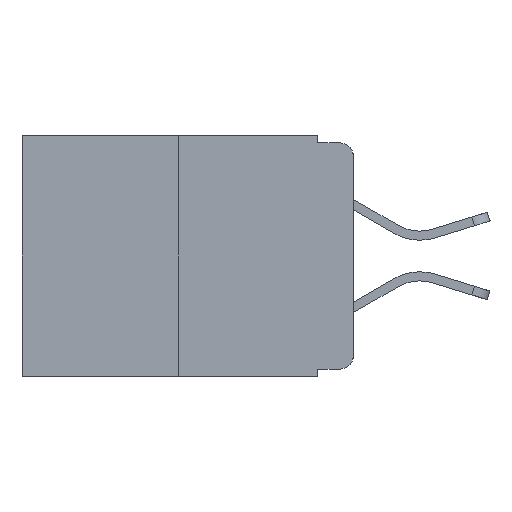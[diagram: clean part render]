
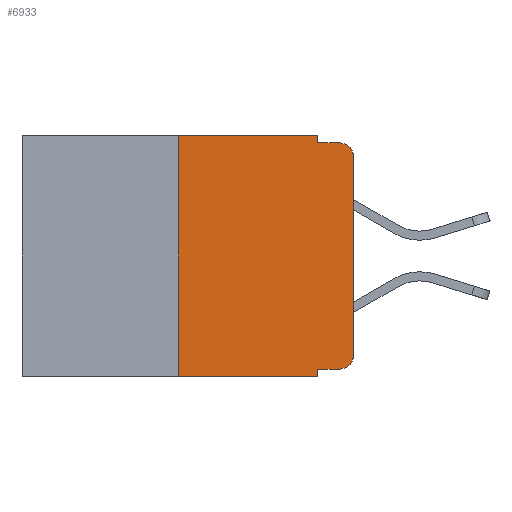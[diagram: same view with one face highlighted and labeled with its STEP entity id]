
A CAD part, left-side view. The second image highlights one B-rep face of the part: STEP entity #6933.
In plain terms, the highlighted planar face has unit normal (-1, 0, 0).
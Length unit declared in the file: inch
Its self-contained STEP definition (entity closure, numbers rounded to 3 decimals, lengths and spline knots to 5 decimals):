
#56 = ORIENTED_EDGE ( 'NONE', *, *, #13089, .T. ) ;
#123 = CARTESIAN_POINT ( 'NONE',  ( 0., 0.051, 0. ) ) ;
#607 = CARTESIAN_POINT ( 'NONE',  ( 0., 0.051, -0.01 ) ) ;
#1297 = VERTEX_POINT ( 'NONE', #15074 ) ;
#1436 = FACE_OUTER_BOUND ( 'NONE', #13858, .T. ) ;
#2048 = EDGE_CURVE ( 'NONE', #14311, #5021, #21147, .T. ) ;
#2507 = ORIENTED_EDGE ( 'NONE', *, *, #4083, .F. ) ;
#2762 = VECTOR ( 'NONE', #11772, 39.37008 ) ;
#3166 = DIRECTION ( 'NONE',  ( 0., -1., 0. ) ) ;
#3186 = EDGE_CURVE ( 'NONE', #1297, #5021, #16227, .T. ) ;
#3219 = ORIENTED_EDGE ( 'NONE', *, *, #9746, .F. ) ;
#3296 = VECTOR ( 'NONE', #3166, 39.37008 ) ;
#3500 = EDGE_CURVE ( 'NONE', #12253, #11377, #20334, .T. ) ;
#3639 = EDGE_CURVE ( 'NONE', #8644, #14191, #11302, .T. ) ;
#3788 = CARTESIAN_POINT ( 'NONE',  ( 0., 0., 0. ) ) ;
#3923 = CARTESIAN_POINT ( 'NONE',  ( 0., 0.051, -0.01 ) ) ;
#4083 = EDGE_CURVE ( 'NONE', #14311, #12253, #13909, .T. ) ;
#4206 = EDGE_CURVE ( 'NONE', #1297, #5745, #5074, .T. ) ;
#4290 = ORIENTED_EDGE ( 'NONE', *, *, #3639, .T. ) ;
#4428 = EDGE_CURVE ( 'NONE', #13529, #14191, #20040, .T. ) ;
#4729 = AXIS2_PLACEMENT_3D ( 'NONE', #18329, #4995, #8584 ) ;
#4995 = DIRECTION ( 'NONE',  ( -1., 0., 0. ) ) ;
#5021 = VERTEX_POINT ( 'NONE', #17077 ) ;
#5074 = LINE ( 'NONE', #17989, #17493 ) ;
#5465 = CARTESIAN_POINT ( 'NONE',  ( 0., 0.02, -0.03 ) ) ;
#5649 = ORIENTED_EDGE ( 'NONE', *, *, #3186, .F. ) ;
#5745 = VERTEX_POINT ( 'NONE', #20886 ) ;
#6933 = ADVANCED_FACE ( 'NONE', ( #1436 ), #10618, .F. ) ;
#6961 = CARTESIAN_POINT ( 'NONE',  ( 0., 0.051, 0. ) ) ;
#6985 = DIRECTION ( 'NONE',  ( 0., 0., 1. ) ) ;
#7328 = CARTESIAN_POINT ( 'NONE',  ( 0., 0.473, -0.343 ) ) ;
#7394 = CIRCLE ( 'NONE', #4729, 0.02 ) ;
#8537 = DIRECTION ( 'NONE',  ( 1., 0., 0. ) ) ;
#8584 = DIRECTION ( 'NONE',  ( 0., 0., -1. ) ) ;
#8644 = VERTEX_POINT ( 'NONE', #13915 ) ;
#9286 = VECTOR ( 'NONE', #10568, 39.37008 ) ;
#9569 = VECTOR ( 'NONE', #6985, 39.37008 ) ;
#9746 = EDGE_CURVE ( 'NONE', #11377, #13529, #17118, .T. ) ;
#10413 = ORIENTED_EDGE ( 'NONE', *, *, #4206, .T. ) ;
#10568 = DIRECTION ( 'NONE',  ( 0., -1., 0. ) ) ;
#10618 = PLANE ( 'NONE',  #13436 ) ;
#11301 = ORIENTED_EDGE ( 'NONE', *, *, #3500, .F. ) ;
#11302 = CIRCLE ( 'NONE', #16244, 0.02 ) ;
#11377 = VERTEX_POINT ( 'NONE', #6961 ) ;
#11388 = VECTOR ( 'NONE', #17624, 39.37008 ) ;
#11772 = DIRECTION ( 'NONE',  ( 0., 0., -1. ) ) ;
#11904 = CARTESIAN_POINT ( 'NONE',  ( 0., 0.02, -0.01 ) ) ;
#12173 = DIRECTION ( 'NONE',  ( 0., -1., 0. ) ) ;
#12253 = VERTEX_POINT ( 'NONE', #14632 ) ;
#12328 = VECTOR ( 'NONE', #19517, 39.37008 ) ;
#12486 = CARTESIAN_POINT ( 'NONE',  ( 0., 0., -0.313 ) ) ;
#12581 = DIRECTION ( 'NONE',  ( -1., 0., 0. ) ) ;
#12709 = CARTESIAN_POINT ( 'NONE',  ( 0., 0.051, 0. ) ) ;
#13089 = EDGE_CURVE ( 'NONE', #5745, #16163, #7394, .T. ) ;
#13268 = DIRECTION ( 'NONE',  ( 0., -1., 0. ) ) ;
#13381 = VECTOR ( 'NONE', #12173, 39.37008 ) ;
#13436 = AXIS2_PLACEMENT_3D ( 'NONE', #16791, #8537, #20093 ) ;
#13529 = VERTEX_POINT ( 'NONE', #3923 ) ;
#13756 = ORIENTED_EDGE ( 'NONE', *, *, #4428, .F. ) ;
#13858 = EDGE_LOOP ( 'NONE', ( #21193, #4290, #13756, #3219, #11301, #2507, #15617, #5649, #10413, #56 ) ) ;
#13909 = LINE ( 'NONE', #16063, #12328 ) ;
#13915 = CARTESIAN_POINT ( 'NONE',  ( 0., 0., -0.03 ) ) ;
#14189 = DIRECTION ( 'NONE',  ( 0., 0., -1. ) ) ;
#14191 = VERTEX_POINT ( 'NONE', #11904 ) ;
#14311 = VERTEX_POINT ( 'NONE', #17654 ) ;
#14632 = CARTESIAN_POINT ( 'NONE',  ( 0., 0.25, 0. ) ) ;
#15074 = CARTESIAN_POINT ( 'NONE',  ( 0., 0.051, -0.333 ) ) ;
#15617 = ORIENTED_EDGE ( 'NONE', *, *, #2048, .T. ) ;
#16063 = CARTESIAN_POINT ( 'NONE',  ( 0., 0.25, 0. ) ) ;
#16163 = VERTEX_POINT ( 'NONE', #12486 ) ;
#16227 = LINE ( 'NONE', #123, #2762 ) ;
#16244 = AXIS2_PLACEMENT_3D ( 'NONE', #5465, #12581, #14189 ) ;
#16791 = CARTESIAN_POINT ( 'NONE',  ( 0., 0.473, 0. ) ) ;
#16801 = LINE ( 'NONE', #3788, #9569 ) ;
#17077 = CARTESIAN_POINT ( 'NONE',  ( 0., 0.051, -0.343 ) ) ;
#17118 = LINE ( 'NONE', #12709, #11388 ) ;
#17493 = VECTOR ( 'NONE', #13268, 39.37008 ) ;
#17581 = EDGE_CURVE ( 'NONE', #16163, #8644, #16801, .T. ) ;
#17624 = DIRECTION ( 'NONE',  ( 0., 0., -1. ) ) ;
#17654 = CARTESIAN_POINT ( 'NONE',  ( 0., 0.25, -0.343 ) ) ;
#17920 = CARTESIAN_POINT ( 'NONE',  ( 0., 0.473, 0. ) ) ;
#17989 = CARTESIAN_POINT ( 'NONE',  ( 0., 0.051, -0.333 ) ) ;
#18329 = CARTESIAN_POINT ( 'NONE',  ( 0., 0.02, -0.313 ) ) ;
#19517 = DIRECTION ( 'NONE',  ( 0., 0., 1. ) ) ;
#20040 = LINE ( 'NONE', #607, #13381 ) ;
#20093 = DIRECTION ( 'NONE',  ( 0., 0., -1. ) ) ;
#20334 = LINE ( 'NONE', #17920, #3296 ) ;
#20886 = CARTESIAN_POINT ( 'NONE',  ( 0., 0.02, -0.333 ) ) ;
#21147 = LINE ( 'NONE', #7328, #9286 ) ;
#21193 = ORIENTED_EDGE ( 'NONE', *, *, #17581, .T. ) ;
